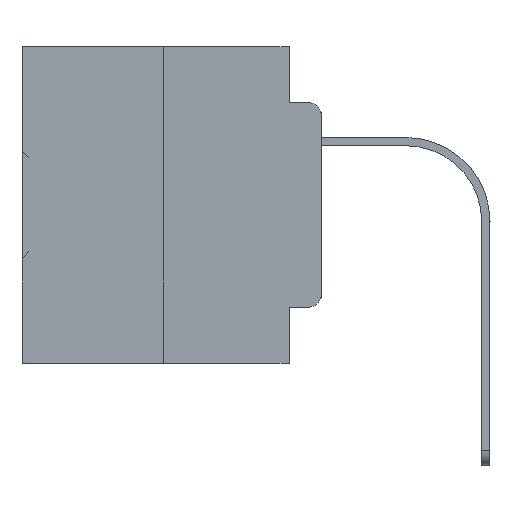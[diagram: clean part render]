
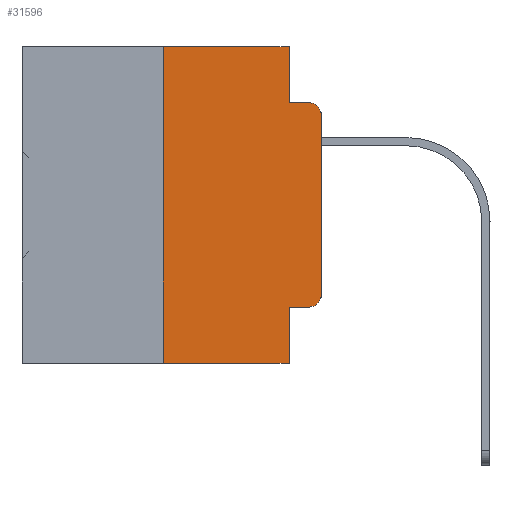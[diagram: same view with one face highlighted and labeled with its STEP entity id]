
A CAD part, left-side view. The second image highlights one B-rep face of the part: STEP entity #31596.
In plain terms, the highlighted planar face has unit normal (-1, 0, 0).
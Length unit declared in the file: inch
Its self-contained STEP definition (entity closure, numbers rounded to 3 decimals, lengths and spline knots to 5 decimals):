
#178 = VERTEX_POINT ( 'NONE', #946 ) ;
#525 = AXIS2_PLACEMENT_3D ( 'NONE', #28881, #3332, #34645 ) ;
#946 = CARTESIAN_POINT ( 'NONE',  ( 0., 0.051, -0.4115 ) ) ;
#1506 = CARTESIAN_POINT ( 'NONE',  ( 0., 0.051, -0.0885 ) ) ;
#2342 = CARTESIAN_POINT ( 'NONE',  ( 0., 0.25, 0. ) ) ;
#2376 = VERTEX_POINT ( 'NONE', #22447 ) ;
#2719 = LINE ( 'NONE', #34389, #17249 ) ;
#2890 = ORIENTED_EDGE ( 'NONE', *, *, #7241, .T. ) ;
#3225 = ORIENTED_EDGE ( 'NONE', *, *, #35114, .F. ) ;
#3332 = DIRECTION ( 'NONE',  ( -1., 0., 0. ) ) ;
#3608 = DIRECTION ( 'NONE',  ( 0., 0., -1. ) ) ;
#3637 = VERTEX_POINT ( 'NONE', #3707 ) ;
#3707 = CARTESIAN_POINT ( 'NONE',  ( 0., 0.051, -0.5 ) ) ;
#4674 = VECTOR ( 'NONE', #36629, 39.37008 ) ;
#4894 = VERTEX_POINT ( 'NONE', #9692 ) ;
#5324 = LINE ( 'NONE', #2342, #35842 ) ;
#5459 = DIRECTION ( 'NONE',  ( 0., 0., -1. ) ) ;
#5818 = DIRECTION ( 'NONE',  ( 1., 0., 0. ) ) ;
#6064 = ORIENTED_EDGE ( 'NONE', *, *, #13018, .F. ) ;
#6199 = EDGE_LOOP ( 'NONE', ( #24522, #22685, #14945, #9034, #3225, #20631, #7999, #6064, #2890, #21634 ) ) ;
#6307 = VECTOR ( 'NONE', #8081, 39.37008 ) ;
#6914 = VERTEX_POINT ( 'NONE', #12977 ) ;
#7241 = EDGE_CURVE ( 'NONE', #178, #19475, #34023, .T. ) ;
#7999 = ORIENTED_EDGE ( 'NONE', *, *, #23968, .T. ) ;
#8081 = DIRECTION ( 'NONE',  ( 0., 0., -1. ) ) ;
#8751 = AXIS2_PLACEMENT_3D ( 'NONE', #28740, #5818, #5459 ) ;
#8790 = PLANE ( 'NONE',  #8751 ) ;
#9034 = ORIENTED_EDGE ( 'NONE', *, *, #21366, .F. ) ;
#9220 = DIRECTION ( 'NONE',  ( -1., 0., 0. ) ) ;
#9452 = DIRECTION ( 'NONE',  ( 0., -1., 0. ) ) ;
#9494 = CARTESIAN_POINT ( 'NONE',  ( 0., 0.473, -0.5 ) ) ;
#9692 = CARTESIAN_POINT ( 'NONE',  ( 0., 0., -0.1085 ) ) ;
#11418 = FACE_OUTER_BOUND ( 'NONE', #6199, .T. ) ;
#11461 = DIRECTION ( 'NONE',  ( 0., 0., 1. ) ) ;
#12110 = CARTESIAN_POINT ( 'NONE',  ( 0., 0.25, -0.5 ) ) ;
#12977 = CARTESIAN_POINT ( 'NONE',  ( 0., 0.051, -0.0885 ) ) ;
#13018 = EDGE_CURVE ( 'NONE', #178, #3637, #27847, .T. ) ;
#13849 = EDGE_CURVE ( 'NONE', #2376, #4894, #2719, .T. ) ;
#14051 = EDGE_CURVE ( 'NONE', #19475, #2376, #16644, .T. ) ;
#14089 = DIRECTION ( 'NONE',  ( 0., 0., 1. ) ) ;
#14945 = ORIENTED_EDGE ( 'NONE', *, *, #23060, .F. ) ;
#16644 = CIRCLE ( 'NONE', #22023, 0.02 ) ;
#17249 = VECTOR ( 'NONE', #14089, 39.37008 ) ;
#17585 = VERTEX_POINT ( 'NONE', #29593 ) ;
#18464 = VECTOR ( 'NONE', #35387, 39.37008 ) ;
#19475 = VERTEX_POINT ( 'NONE', #22882 ) ;
#20401 = CARTESIAN_POINT ( 'NONE',  ( 0., 0.051, 0. ) ) ;
#20424 = CARTESIAN_POINT ( 'NONE',  ( 0., 0.02, -0.3915 ) ) ;
#20631 = ORIENTED_EDGE ( 'NONE', *, *, #27733, .F. ) ;
#20796 = CIRCLE ( 'NONE', #525, 0.02 ) ;
#21082 = VECTOR ( 'NONE', #3608, 39.37008 ) ;
#21366 = EDGE_CURVE ( 'NONE', #22207, #6914, #34913, .T. ) ;
#21634 = ORIENTED_EDGE ( 'NONE', *, *, #14051, .T. ) ;
#22004 = VECTOR ( 'NONE', #32836, 39.37008 ) ;
#22023 = AXIS2_PLACEMENT_3D ( 'NONE', #20424, #9220, #32331 ) ;
#22207 = VERTEX_POINT ( 'NONE', #29607 ) ;
#22447 = CARTESIAN_POINT ( 'NONE',  ( 0., 0., -0.3915 ) ) ;
#22685 = ORIENTED_EDGE ( 'NONE', *, *, #23368, .T. ) ;
#22882 = CARTESIAN_POINT ( 'NONE',  ( 0., 0.02, -0.4115 ) ) ;
#23060 = EDGE_CURVE ( 'NONE', #6914, #33312, #33390, .T. ) ;
#23368 = EDGE_CURVE ( 'NONE', #4894, #33312, #20796, .T. ) ;
#23968 = EDGE_CURVE ( 'NONE', #29711, #3637, #35017, .T. ) ;
#23993 = LINE ( 'NONE', #35346, #24055 ) ;
#24055 = VECTOR ( 'NONE', #9452, 39.37008 ) ;
#24522 = ORIENTED_EDGE ( 'NONE', *, *, #13849, .T. ) ;
#25287 = CARTESIAN_POINT ( 'NONE',  ( 0., 0.051, -0.4115 ) ) ;
#27733 = EDGE_CURVE ( 'NONE', #29711, #17585, #5324, .T. ) ;
#27847 = LINE ( 'NONE', #28585, #6307 ) ;
#28155 = CARTESIAN_POINT ( 'NONE',  ( 0., 0.02, -0.0885 ) ) ;
#28585 = CARTESIAN_POINT ( 'NONE',  ( 0., 0.051, 0. ) ) ;
#28740 = CARTESIAN_POINT ( 'NONE',  ( 0., 0.473, 0. ) ) ;
#28881 = CARTESIAN_POINT ( 'NONE',  ( 0., 0.02, -0.1085 ) ) ;
#29593 = CARTESIAN_POINT ( 'NONE',  ( 0., 0.25, 0. ) ) ;
#29607 = CARTESIAN_POINT ( 'NONE',  ( 0., 0.051, 0. ) ) ;
#29711 = VERTEX_POINT ( 'NONE', #12110 ) ;
#31596 = ADVANCED_FACE ( 'NONE', ( #11418 ), #8790, .F. ) ;
#32331 = DIRECTION ( 'NONE',  ( 0., 0., -1. ) ) ;
#32836 = DIRECTION ( 'NONE',  ( 0., -1., 0. ) ) ;
#33312 = VERTEX_POINT ( 'NONE', #28155 ) ;
#33390 = LINE ( 'NONE', #1506, #22004 ) ;
#34023 = LINE ( 'NONE', #25287, #4674 ) ;
#34389 = CARTESIAN_POINT ( 'NONE',  ( 0., 0., 0. ) ) ;
#34645 = DIRECTION ( 'NONE',  ( 0., 0., -1. ) ) ;
#34913 = LINE ( 'NONE', #20401, #21082 ) ;
#35017 = LINE ( 'NONE', #9494, #18464 ) ;
#35114 = EDGE_CURVE ( 'NONE', #17585, #22207, #23993, .T. ) ;
#35346 = CARTESIAN_POINT ( 'NONE',  ( 0., 0.473, 0. ) ) ;
#35387 = DIRECTION ( 'NONE',  ( 0., -1., 0. ) ) ;
#35842 = VECTOR ( 'NONE', #11461, 39.37008 ) ;
#36629 = DIRECTION ( 'NONE',  ( 0., -1., 0. ) ) ;
